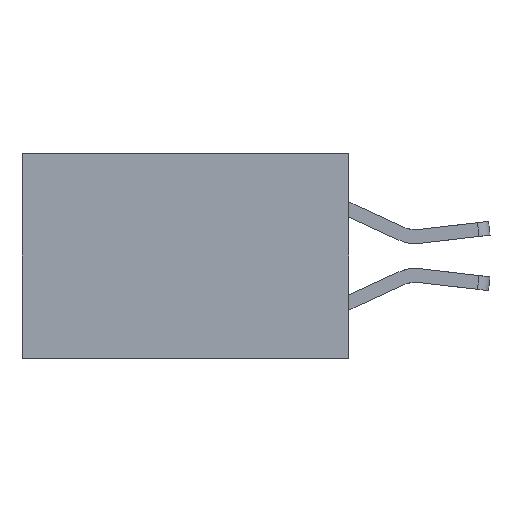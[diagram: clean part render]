
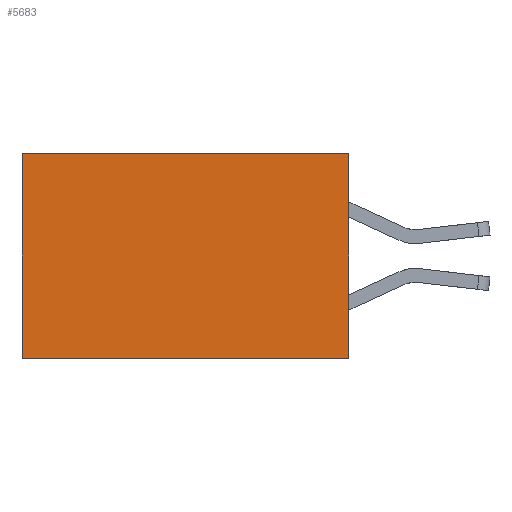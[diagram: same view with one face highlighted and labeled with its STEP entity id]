
A CAD part, left-side view. The second image highlights one B-rep face of the part: STEP entity #5683.
In plain terms, the highlighted planar face has unit normal (-1, 0, 0).
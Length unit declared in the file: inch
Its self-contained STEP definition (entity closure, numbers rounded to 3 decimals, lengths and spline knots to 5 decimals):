
#217 = DIRECTION ( 'NONE',  ( 0., 0., -1. ) ) ;
#263 = EDGE_CURVE ( 'NONE', #4220, #282, #8059, .T. ) ;
#282 = VERTEX_POINT ( 'NONE', #610 ) ;
#311 = DIRECTION ( 'NONE',  ( 1., 0., 0. ) ) ;
#552 = DIRECTION ( 'NONE',  ( 0., 1., 0. ) ) ;
#610 = CARTESIAN_POINT ( 'NONE',  ( 0.277, 0.59, -0.37 ) ) ;
#1023 = LINE ( 'NONE', #1837, #2856 ) ;
#1290 = AXIS2_PLACEMENT_3D ( 'NONE', #4412, #311, #5062 ) ;
#1301 = EDGE_CURVE ( 'NONE', #1679, #282, #5923, .T. ) ;
#1404 = EDGE_CURVE ( 'NONE', #1787, #1679, #7013, .T. ) ;
#1624 = CARTESIAN_POINT ( 'NONE',  ( 0.277, 0.59, -0.37 ) ) ;
#1679 = VERTEX_POINT ( 'NONE', #5270 ) ;
#1698 = PLANE ( 'NONE',  #1290 ) ;
#1787 = VERTEX_POINT ( 'NONE', #2750 ) ;
#1837 = CARTESIAN_POINT ( 'NONE',  ( 0.277, 0., 0. ) ) ;
#1949 = CARTESIAN_POINT ( 'NONE',  ( 0.277, 0., -0.37 ) ) ;
#2525 = DIRECTION ( 'NONE',  ( 0., 0., -1. ) ) ;
#2750 = CARTESIAN_POINT ( 'NONE',  ( 0.277, 0., 0. ) ) ;
#2856 = VECTOR ( 'NONE', #4480, 39.37008 ) ;
#3153 = FACE_OUTER_BOUND ( 'NONE', #5866, .T. ) ;
#3351 = ORIENTED_EDGE ( 'NONE', *, *, #263, .T. ) ;
#3361 = ORIENTED_EDGE ( 'NONE', *, *, #1301, .F. ) ;
#3411 = ORIENTED_EDGE ( 'NONE', *, *, #1404, .F. ) ;
#3452 = ORIENTED_EDGE ( 'NONE', *, *, #5082, .T. ) ;
#4220 = VERTEX_POINT ( 'NONE', #6899 ) ;
#4412 = CARTESIAN_POINT ( 'NONE',  ( 0.277, 0., -0.37 ) ) ;
#4480 = DIRECTION ( 'NONE',  ( 0., 1., 0. ) ) ;
#5062 = DIRECTION ( 'NONE',  ( 0., 0., -1. ) ) ;
#5082 = EDGE_CURVE ( 'NONE', #1787, #4220, #1023, .T. ) ;
#5270 = CARTESIAN_POINT ( 'NONE',  ( 0.277, 0., -0.37 ) ) ;
#5683 = ADVANCED_FACE ( 'NONE', ( #3153 ), #1698, .F. ) ;
#5866 = EDGE_LOOP ( 'NONE', ( #3351, #3361, #3411, #3452 ) ) ;
#5923 = LINE ( 'NONE', #1949, #6112 ) ;
#6112 = VECTOR ( 'NONE', #552, 39.37008 ) ;
#6571 = CARTESIAN_POINT ( 'NONE',  ( 0.277, 0., -0.37 ) ) ;
#6629 = VECTOR ( 'NONE', #217, 39.37008 ) ;
#6899 = CARTESIAN_POINT ( 'NONE',  ( 0.277, 0.59, 0. ) ) ;
#7013 = LINE ( 'NONE', #6571, #8219 ) ;
#8059 = LINE ( 'NONE', #1624, #6629 ) ;
#8219 = VECTOR ( 'NONE', #2525, 39.37008 ) ;
